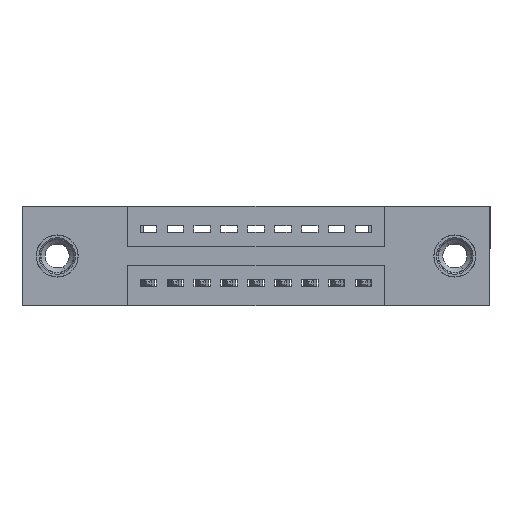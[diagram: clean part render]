
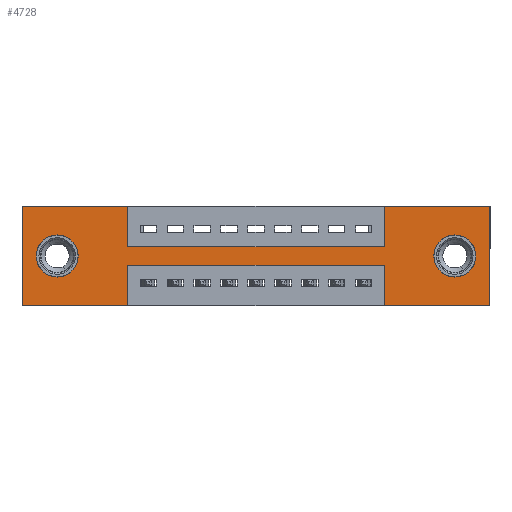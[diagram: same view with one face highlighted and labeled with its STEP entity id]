
A CAD part, front view. The second image highlights one B-rep face of the part: STEP entity #4728.
In plain terms, the highlighted planar face has unit normal (0, -1, 0).
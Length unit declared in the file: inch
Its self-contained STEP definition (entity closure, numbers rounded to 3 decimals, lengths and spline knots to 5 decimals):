
#25 = ORIENTED_EDGE ( 'NONE', *, *, #11837, .F. ) ;
#179 = DIRECTION ( 'NONE',  ( 1., 0., 0. ) ) ;
#234 = ORIENTED_EDGE ( 'NONE', *, *, #4874, .F. ) ;
#368 = FACE_BOUND ( 'NONE', #1507, .T. ) ;
#761 = CARTESIAN_POINT ( 'NONE',  ( 0.3925, 0., -0.22 ) ) ;
#874 = DIRECTION ( 'NONE',  ( 0., 0., 1. ) ) ;
#1101 = VERTEX_POINT ( 'NONE', #9722 ) ;
#1457 = EDGE_CURVE ( 'NONE', #2960, #9400, #10035, .T. ) ;
#1458 = CARTESIAN_POINT ( 'NONE',  ( 0.13, 0., -0.107 ) ) ;
#1507 = EDGE_LOOP ( 'NONE', ( #11931, #8327 ) ) ;
#1534 = PLANE ( 'NONE',  #5800 ) ;
#1688 = DIRECTION ( 'NONE',  ( 0., -1., 0. ) ) ;
#1717 = VERTEX_POINT ( 'NONE', #8675 ) ;
#1718 = VERTEX_POINT ( 'NONE', #11309 ) ;
#1942 = VECTOR ( 'NONE', #7895, 39.37008 ) ;
#2318 = CIRCLE ( 'NONE', #3759, 0.078 ) ;
#2354 = VECTOR ( 'NONE', #14647, 39.37008 ) ;
#2440 = DIRECTION ( 'NONE',  ( 0., 0., -1. ) ) ;
#2487 = FACE_BOUND ( 'NONE', #14820, .T. ) ;
#2751 = CARTESIAN_POINT ( 'NONE',  ( 0., 0., -0.37 ) ) ;
#2960 = VERTEX_POINT ( 'NONE', #8456 ) ;
#3071 = DIRECTION ( 'NONE',  ( -1., 0., 0. ) ) ;
#3229 = CARTESIAN_POINT ( 'NONE',  ( 0.3925, 0., -0.22 ) ) ;
#3281 = CARTESIAN_POINT ( 'NONE',  ( 1.3425, 0., -0.37 ) ) ;
#3296 = DIRECTION ( 'NONE',  ( 0., 0., 1. ) ) ;
#3571 = VECTOR ( 'NONE', #5617, 39.37008 ) ;
#3593 = VERTEX_POINT ( 'NONE', #11553 ) ;
#3759 = AXIS2_PLACEMENT_3D ( 'NONE', #10556, #15593, #5735 ) ;
#3762 = VERTEX_POINT ( 'NONE', #761 ) ;
#3970 = EDGE_CURVE ( 'NONE', #15690, #13634, #6710, .T. ) ;
#3997 = VECTOR ( 'NONE', #3071, 39.37008 ) ;
#4514 = CARTESIAN_POINT ( 'NONE',  ( 1.735, 0., -0.37 ) ) ;
#4593 = VECTOR ( 'NONE', #12154, 39.37008 ) ;
#4728 = ADVANCED_FACE ( 'NONE', ( #368, #2487, #6411 ), #1534, .T. ) ;
#4746 = ORIENTED_EDGE ( 'NONE', *, *, #13456, .F. ) ;
#4874 = EDGE_CURVE ( 'NONE', #12793, #6571, #10549, .T. ) ;
#4884 = DIRECTION ( 'NONE',  ( 0., 1., 0. ) ) ;
#5002 = DIRECTION ( 'NONE',  ( 0., 1., 0. ) ) ;
#5091 = CARTESIAN_POINT ( 'NONE',  ( 0., 0., 0. ) ) ;
#5486 = DIRECTION ( 'NONE',  ( 0., 0., -1. ) ) ;
#5617 = DIRECTION ( 'NONE',  ( -1., 0., 0. ) ) ;
#5702 = CARTESIAN_POINT ( 'NONE',  ( 0., 0., -0.37 ) ) ;
#5735 = DIRECTION ( 'NONE',  ( 0., 0., -1. ) ) ;
#5800 = AXIS2_PLACEMENT_3D ( 'NONE', #2751, #1688, #2440 ) ;
#5877 = DIRECTION ( 'NONE',  ( 0., 1., 0. ) ) ;
#5935 = CARTESIAN_POINT ( 'NONE',  ( 0., 0., 0. ) ) ;
#5998 = EDGE_CURVE ( 'NONE', #3593, #3762, #14493, .T. ) ;
#6087 = DIRECTION ( 'NONE',  ( 0., 0., -1. ) ) ;
#6131 = EDGE_CURVE ( 'NONE', #1718, #7571, #2318, .T. ) ;
#6279 = ORIENTED_EDGE ( 'NONE', *, *, #15845, .T. ) ;
#6309 = ORIENTED_EDGE ( 'NONE', *, *, #6626, .F. ) ;
#6411 = FACE_OUTER_BOUND ( 'NONE', #7405, .T. ) ;
#6445 = ORIENTED_EDGE ( 'NONE', *, *, #14279, .F. ) ;
#6558 = ORIENTED_EDGE ( 'NONE', *, *, #1457, .F. ) ;
#6570 = EDGE_CURVE ( 'NONE', #13272, #10283, #6872, .T. ) ;
#6571 = VERTEX_POINT ( 'NONE', #14151 ) ;
#6626 = EDGE_CURVE ( 'NONE', #6571, #1717, #13262, .T. ) ;
#6710 = LINE ( 'NONE', #12529, #11738 ) ;
#6768 = ORIENTED_EDGE ( 'NONE', *, *, #12608, .F. ) ;
#6871 = CARTESIAN_POINT ( 'NONE',  ( 0.13, 0., -0.185 ) ) ;
#6872 = CIRCLE ( 'NONE', #14222, 0.078 ) ;
#6887 = DIRECTION ( 'NONE',  ( 0., 0., 1. ) ) ;
#6921 = LINE ( 'NONE', #11380, #13535 ) ;
#6925 = VERTEX_POINT ( 'NONE', #5091 ) ;
#7241 = EDGE_CURVE ( 'NONE', #7571, #1718, #11314, .T. ) ;
#7243 = LINE ( 'NONE', #12776, #3997 ) ;
#7304 = EDGE_CURVE ( 'NONE', #13841, #1101, #7243, .T. ) ;
#7405 = EDGE_LOOP ( 'NONE', ( #9504, #11470, #6445, #12451, #11559, #7548, #25, #6309, #234, #4746, #6768, #6558 ) ) ;
#7548 = ORIENTED_EDGE ( 'NONE', *, *, #3970, .F. ) ;
#7571 = VERTEX_POINT ( 'NONE', #9358 ) ;
#7895 = DIRECTION ( 'NONE',  ( -1., 0., 0. ) ) ;
#8003 = VECTOR ( 'NONE', #14555, 39.37008 ) ;
#8240 = VECTOR ( 'NONE', #3296, 39.37008 ) ;
#8242 = VECTOR ( 'NONE', #5486, 39.37008 ) ;
#8327 = ORIENTED_EDGE ( 'NONE', *, *, #6131, .T. ) ;
#8456 = CARTESIAN_POINT ( 'NONE',  ( 0.3925, 0., -0.37 ) ) ;
#8509 = CARTESIAN_POINT ( 'NONE',  ( 0.13, 0., -0.185 ) ) ;
#8675 = CARTESIAN_POINT ( 'NONE',  ( 1.3425, 0., -0.15 ) ) ;
#9016 = DIRECTION ( 'NONE',  ( 0., 0., -1. ) ) ;
#9228 = VECTOR ( 'NONE', #6887, 39.37008 ) ;
#9293 = CARTESIAN_POINT ( 'NONE',  ( 0., 0., 0. ) ) ;
#9358 = CARTESIAN_POINT ( 'NONE',  ( 1.605, 0., -0.107 ) ) ;
#9400 = VERTEX_POINT ( 'NONE', #5702 ) ;
#9422 = DIRECTION ( 'NONE',  ( 0., 0., 1. ) ) ;
#9504 = ORIENTED_EDGE ( 'NONE', *, *, #13643, .F. ) ;
#9722 = CARTESIAN_POINT ( 'NONE',  ( 1.3425, 0., -0.37 ) ) ;
#10035 = LINE ( 'NONE', #11808, #3571 ) ;
#10283 = VERTEX_POINT ( 'NONE', #15623 ) ;
#10319 = CIRCLE ( 'NONE', #11963, 0.078 ) ;
#10539 = CARTESIAN_POINT ( 'NONE',  ( 0.3925, 0., 0. ) ) ;
#10549 = LINE ( 'NONE', #10539, #4593 ) ;
#10556 = CARTESIAN_POINT ( 'NONE',  ( 1.605, 0., -0.185 ) ) ;
#10766 = VECTOR ( 'NONE', #874, 39.37008 ) ;
#10884 = CARTESIAN_POINT ( 'NONE',  ( 0.3925, 0., -0.15 ) ) ;
#11309 = CARTESIAN_POINT ( 'NONE',  ( 1.605, 0., -0.263 ) ) ;
#11314 = CIRCLE ( 'NONE', #14951, 0.078 ) ;
#11380 = CARTESIAN_POINT ( 'NONE',  ( 1.735, 0., 0. ) ) ;
#11470 = ORIENTED_EDGE ( 'NONE', *, *, #5998, .F. ) ;
#11553 = CARTESIAN_POINT ( 'NONE',  ( 1.3425, 0., -0.22 ) ) ;
#11559 = ORIENTED_EDGE ( 'NONE', *, *, #11591, .F. ) ;
#11591 = EDGE_CURVE ( 'NONE', #13634, #13841, #6921, .T. ) ;
#11738 = VECTOR ( 'NONE', #179, 39.37008 ) ;
#11808 = CARTESIAN_POINT ( 'NONE',  ( 0., 0., -0.37 ) ) ;
#11837 = EDGE_CURVE ( 'NONE', #1717, #15690, #14509, .T. ) ;
#11931 = ORIENTED_EDGE ( 'NONE', *, *, #7241, .T. ) ;
#11963 = AXIS2_PLACEMENT_3D ( 'NONE', #6871, #5877, #9422 ) ;
#11982 = LINE ( 'NONE', #9293, #9228 ) ;
#12154 = DIRECTION ( 'NONE',  ( 0., 0., -1. ) ) ;
#12451 = ORIENTED_EDGE ( 'NONE', *, *, #7304, .F. ) ;
#12529 = CARTESIAN_POINT ( 'NONE',  ( 0., 0., 0. ) ) ;
#12608 = EDGE_CURVE ( 'NONE', #9400, #6925, #11982, .T. ) ;
#12712 = ORIENTED_EDGE ( 'NONE', *, *, #6570, .T. ) ;
#12776 = CARTESIAN_POINT ( 'NONE',  ( 0., 0., -0.37 ) ) ;
#12793 = VERTEX_POINT ( 'NONE', #13813 ) ;
#12851 = CARTESIAN_POINT ( 'NONE',  ( 0.3925, 0., -0.37 ) ) ;
#13262 = LINE ( 'NONE', #10884, #8003 ) ;
#13272 = VERTEX_POINT ( 'NONE', #1458 ) ;
#13456 = EDGE_CURVE ( 'NONE', #6925, #12793, #14510, .T. ) ;
#13535 = VECTOR ( 'NONE', #9016, 39.37008 ) ;
#13602 = DIRECTION ( 'NONE',  ( 0., 0., 1. ) ) ;
#13634 = VERTEX_POINT ( 'NONE', #14265 ) ;
#13643 = EDGE_CURVE ( 'NONE', #3762, #2960, #13914, .T. ) ;
#13813 = CARTESIAN_POINT ( 'NONE',  ( 0.3925, 0., 0. ) ) ;
#13841 = VERTEX_POINT ( 'NONE', #4514 ) ;
#13914 = LINE ( 'NONE', #12851, #8242 ) ;
#14093 = LINE ( 'NONE', #3281, #10766 ) ;
#14151 = CARTESIAN_POINT ( 'NONE',  ( 0.3925, 0., -0.15 ) ) ;
#14222 = AXIS2_PLACEMENT_3D ( 'NONE', #8509, #4884, #13602 ) ;
#14265 = CARTESIAN_POINT ( 'NONE',  ( 1.735, 0., 0. ) ) ;
#14279 = EDGE_CURVE ( 'NONE', #1101, #3593, #14093, .T. ) ;
#14493 = LINE ( 'NONE', #3229, #1942 ) ;
#14509 = LINE ( 'NONE', #15720, #8240 ) ;
#14510 = LINE ( 'NONE', #5935, #2354 ) ;
#14555 = DIRECTION ( 'NONE',  ( 1., 0., 0. ) ) ;
#14647 = DIRECTION ( 'NONE',  ( 1., 0., 0. ) ) ;
#14815 = CARTESIAN_POINT ( 'NONE',  ( 1.605, 0., -0.185 ) ) ;
#14820 = EDGE_LOOP ( 'NONE', ( #12712, #6279 ) ) ;
#14951 = AXIS2_PLACEMENT_3D ( 'NONE', #14815, #5002, #6087 ) ;
#15220 = CARTESIAN_POINT ( 'NONE',  ( 1.3425, 0., 0. ) ) ;
#15593 = DIRECTION ( 'NONE',  ( 0., 1., 0. ) ) ;
#15623 = CARTESIAN_POINT ( 'NONE',  ( 0.13, 0., -0.263 ) ) ;
#15690 = VERTEX_POINT ( 'NONE', #15220 ) ;
#15720 = CARTESIAN_POINT ( 'NONE',  ( 1.3425, 0., 0. ) ) ;
#15845 = EDGE_CURVE ( 'NONE', #10283, #13272, #10319, .T. ) ;
